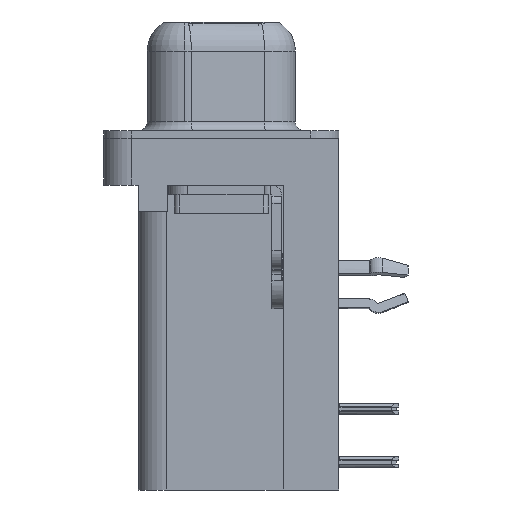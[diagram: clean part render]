
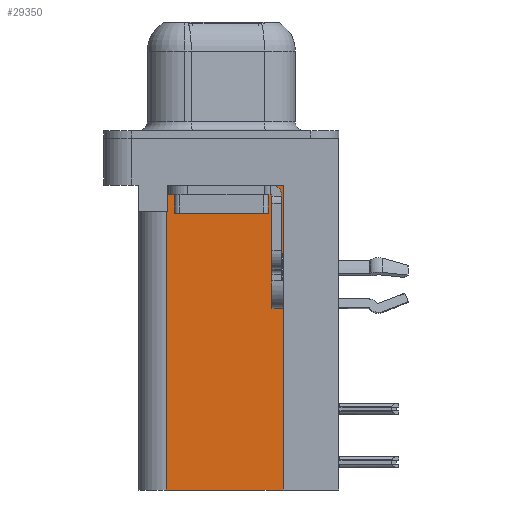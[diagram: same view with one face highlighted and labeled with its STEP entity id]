
A CAD part, left-side view. The second image highlights one B-rep face of the part: STEP entity #29350.
In plain terms, the highlighted planar face has unit normal (-1, 0, 0).
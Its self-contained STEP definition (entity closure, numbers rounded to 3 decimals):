
#481 = AXIS2_PLACEMENT_3D ( 'NONE', #22284, #1157, #17732 ) ;
#602 = EDGE_CURVE ( 'NONE', #11873, #9342, #27453, .T. ) ;
#681 = LINE ( 'NONE', #2174, #795 ) ;
#795 = VECTOR ( 'NONE', #16412, 1000. ) ;
#1157 = DIRECTION ( 'NONE',  ( 1., 0., 0. ) ) ;
#1491 = ORIENTED_EDGE ( 'NONE', *, *, #17093, .F. ) ;
#1499 = CARTESIAN_POINT ( 'NONE',  ( 3.7, -3.295, -18.76 ) ) ;
#1936 = CARTESIAN_POINT ( 'NONE',  ( 3.7, -3.295, -2.5 ) ) ;
#2172 = EDGE_CURVE ( 'NONE', #11873, #28589, #20620, .T. ) ;
#2174 = CARTESIAN_POINT ( 'NONE',  ( 3.7, 2.925, -18.76 ) ) ;
#4188 = ORIENTED_EDGE ( 'NONE', *, *, #15682, .T. ) ;
#4992 = CARTESIAN_POINT ( 'NONE',  ( 3.7, 2.925, -3.9 ) ) ;
#5110 = FACE_OUTER_BOUND ( 'NONE', #12944, .T. ) ;
#5391 = VECTOR ( 'NONE', #7808, 1000. ) ;
#5622 = LINE ( 'NONE', #12757, #5391 ) ;
#6068 = VERTEX_POINT ( 'NONE', #6985 ) ;
#6985 = CARTESIAN_POINT ( 'NONE',  ( 3.7, 2.895, -2.5 ) ) ;
#6989 = VECTOR ( 'NONE', #13264, 1000. ) ;
#7082 = LINE ( 'NONE', #17965, #6989 ) ;
#7808 = DIRECTION ( 'NONE',  ( 0., 1., 0. ) ) ;
#8557 = ORIENTED_EDGE ( 'NONE', *, *, #8648, .T. ) ;
#8648 = EDGE_CURVE ( 'NONE', #29487, #17871, #18961, .T. ) ;
#9342 = VERTEX_POINT ( 'NONE', #22467 ) ;
#10127 = CARTESIAN_POINT ( 'NONE',  ( 3.7, -3.295, -18.76 ) ) ;
#10347 = DIRECTION ( 'NONE',  ( 0., 0., 1. ) ) ;
#11873 = VERTEX_POINT ( 'NONE', #1499 ) ;
#12293 = DIRECTION ( 'NONE',  ( 0., 1., 0. ) ) ;
#12757 = CARTESIAN_POINT ( 'NONE',  ( 3.7, -3.295, -2.5 ) ) ;
#12944 = EDGE_LOOP ( 'NONE', ( #18465, #4188, #8557, #1491, #19128, #25255 ) ) ;
#13022 = PLANE ( 'NONE',  #481 ) ;
#13264 = DIRECTION ( 'NONE',  ( 0., 0., -1. ) ) ;
#15682 = EDGE_CURVE ( 'NONE', #6068, #29487, #7082, .T. ) ;
#16412 = DIRECTION ( 'NONE',  ( 0., 0., 1. ) ) ;
#17093 = EDGE_CURVE ( 'NONE', #9342, #17871, #681, .T. ) ;
#17732 = DIRECTION ( 'NONE',  ( 0., 1., 0. ) ) ;
#17871 = VERTEX_POINT ( 'NONE', #4992 ) ;
#17965 = CARTESIAN_POINT ( 'NONE',  ( 3.7, 2.895, -3.9 ) ) ;
#18465 = ORIENTED_EDGE ( 'NONE', *, *, #22471, .T. ) ;
#18767 = VECTOR ( 'NONE', #12293, 1000. ) ;
#18961 = LINE ( 'NONE', #26308, #18767 ) ;
#19128 = ORIENTED_EDGE ( 'NONE', *, *, #602, .F. ) ;
#20620 = LINE ( 'NONE', #10127, #20693 ) ;
#20693 = VECTOR ( 'NONE', #10347, 1000. ) ;
#22284 = CARTESIAN_POINT ( 'NONE',  ( 3.7, -3.295, -18.76 ) ) ;
#22467 = CARTESIAN_POINT ( 'NONE',  ( 3.7, 2.925, -18.76 ) ) ;
#22471 = EDGE_CURVE ( 'NONE', #28589, #6068, #5622, .T. ) ;
#25145 = CARTESIAN_POINT ( 'NONE',  ( 3.7, 2.895, -3.9 ) ) ;
#25255 = ORIENTED_EDGE ( 'NONE', *, *, #2172, .T. ) ;
#26308 = CARTESIAN_POINT ( 'NONE',  ( 3.7, 0., -3.9 ) ) ;
#27135 = DIRECTION ( 'NONE',  ( 0., 1., 0. ) ) ;
#27320 = VECTOR ( 'NONE', #27135, 1000. ) ;
#27453 = LINE ( 'NONE', #30216, #27320 ) ;
#28589 = VERTEX_POINT ( 'NONE', #1936 ) ;
#29350 = ADVANCED_FACE ( 'NONE', ( #5110 ), #13022, .F. ) ;
#29487 = VERTEX_POINT ( 'NONE', #25145 ) ;
#30216 = CARTESIAN_POINT ( 'NONE',  ( 3.7, -3.295, -18.76 ) ) ;
